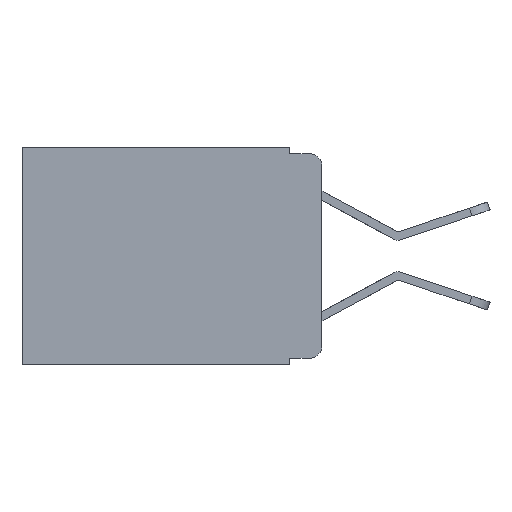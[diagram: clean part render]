
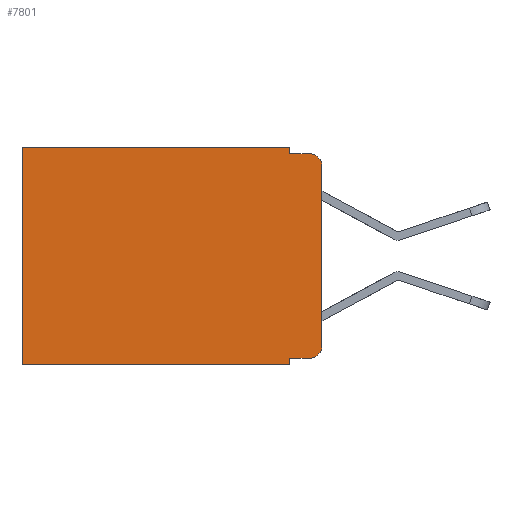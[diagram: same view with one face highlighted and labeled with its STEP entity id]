
A CAD part, left-side view. The second image highlights one B-rep face of the part: STEP entity #7801.
In plain terms, the highlighted planar face has unit normal (-1, 0, 0).
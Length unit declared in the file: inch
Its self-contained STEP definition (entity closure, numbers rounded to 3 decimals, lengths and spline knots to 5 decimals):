
#41 = EDGE_CURVE ( 'NONE', #6747, #13839, #7607, .T. ) ;
#63 = CARTESIAN_POINT ( 'NONE',  ( 0.298, 0.051, -0.01 ) ) ;
#324 = CARTESIAN_POINT ( 'NONE',  ( 0.298, 0.02, -0.333 ) ) ;
#330 = EDGE_LOOP ( 'NONE', ( #10132, #17698, #12927, #10647, #9686, #11313, #15292, #1041, #15936, #714 ) ) ;
#372 = LINE ( 'NONE', #13331, #14365 ) ;
#389 = EDGE_CURVE ( 'NONE', #1333, #15356, #3936, .T. ) ;
#497 = CARTESIAN_POINT ( 'NONE',  ( 0.298, 0.051, -0.343 ) ) ;
#714 = ORIENTED_EDGE ( 'NONE', *, *, #389, .T. ) ;
#875 = VERTEX_POINT ( 'NONE', #497 ) ;
#1041 = ORIENTED_EDGE ( 'NONE', *, *, #13506, .F. ) ;
#1333 = VERTEX_POINT ( 'NONE', #324 ) ;
#1615 = LINE ( 'NONE', #13064, #16016 ) ;
#1883 = LINE ( 'NONE', #7735, #16280 ) ;
#2025 = VECTOR ( 'NONE', #6155, 39.37008 ) ;
#2294 = EDGE_CURVE ( 'NONE', #14530, #1333, #1883, .T. ) ;
#2947 = LINE ( 'NONE', #15879, #2025 ) ;
#3490 = EDGE_CURVE ( 'NONE', #10490, #10364, #11896, .T. ) ;
#3571 = CARTESIAN_POINT ( 'NONE',  ( 0.298, 0., -0.03 ) ) ;
#3912 = VECTOR ( 'NONE', #8870, 39.37008 ) ;
#3936 = CIRCLE ( 'NONE', #10385, 0.02 ) ;
#4143 = VECTOR ( 'NONE', #13033, 39.37008 ) ;
#4738 = DIRECTION ( 'NONE',  ( -1., 0., 0. ) ) ;
#4777 = CARTESIAN_POINT ( 'NONE',  ( 0.298, 0.02, -0.03 ) ) ;
#4855 = CARTESIAN_POINT ( 'NONE',  ( 0.298, 0.473, -0.343 ) ) ;
#5019 = DIRECTION ( 'NONE',  ( 0., 0., -1. ) ) ;
#5023 = CARTESIAN_POINT ( 'NONE',  ( 0.298, 0., -0.313 ) ) ;
#5196 = DIRECTION ( 'NONE',  ( 1., 0., 0. ) ) ;
#6155 = DIRECTION ( 'NONE',  ( 0., 1., 0. ) ) ;
#6409 = CARTESIAN_POINT ( 'NONE',  ( 0.298, 0.473, 0. ) ) ;
#6421 = FACE_OUTER_BOUND ( 'NONE', #330, .T. ) ;
#6747 = VERTEX_POINT ( 'NONE', #14285 ) ;
#7385 = DIRECTION ( 'NONE',  ( 0., 0., -1. ) ) ;
#7607 = LINE ( 'NONE', #10515, #3912 ) ;
#7622 = DIRECTION ( 'NONE',  ( 0., -1., 0. ) ) ;
#7626 = EDGE_CURVE ( 'NONE', #6747, #16490, #2947, .T. ) ;
#7735 = CARTESIAN_POINT ( 'NONE',  ( 0.298, 0.051, -0.333 ) ) ;
#7801 = ADVANCED_FACE ( 'NONE', ( #6421 ), #13512, .F. ) ;
#7842 = LINE ( 'NONE', #8880, #4143 ) ;
#8300 = EDGE_CURVE ( 'NONE', #875, #12266, #16808, .T. ) ;
#8870 = DIRECTION ( 'NONE',  ( 0., 0., -1. ) ) ;
#8880 = CARTESIAN_POINT ( 'NONE',  ( 0.298, 0.051, -0.01 ) ) ;
#9223 = DIRECTION ( 'NONE',  ( 0., 0., -1. ) ) ;
#9313 = LINE ( 'NONE', #6409, #16238 ) ;
#9339 = CARTESIAN_POINT ( 'NONE',  ( 0.298, 0., 0. ) ) ;
#9686 = ORIENTED_EDGE ( 'NONE', *, *, #7626, .T. ) ;
#9743 = CARTESIAN_POINT ( 'NONE',  ( 0.298, 0.473, 0. ) ) ;
#9757 = AXIS2_PLACEMENT_3D ( 'NONE', #9339, #5196, #14919 ) ;
#10132 = ORIENTED_EDGE ( 'NONE', *, *, #15608, .F. ) ;
#10358 = DIRECTION ( 'NONE',  ( -1., 0., 0. ) ) ;
#10364 = VERTEX_POINT ( 'NONE', #11662 ) ;
#10372 = EDGE_CURVE ( 'NONE', #13839, #10364, #7842, .T. ) ;
#10385 = AXIS2_PLACEMENT_3D ( 'NONE', #17068, #10358, #16396 ) ;
#10490 = VERTEX_POINT ( 'NONE', #3571 ) ;
#10515 = CARTESIAN_POINT ( 'NONE',  ( 0.298, 0.051, 0. ) ) ;
#10647 = ORIENTED_EDGE ( 'NONE', *, *, #41, .F. ) ;
#11313 = ORIENTED_EDGE ( 'NONE', *, *, #15384, .T. ) ;
#11662 = CARTESIAN_POINT ( 'NONE',  ( 0.298, 0.02, -0.01 ) ) ;
#11689 = DIRECTION ( 'NONE',  ( 0., 0., -1. ) ) ;
#11896 = CIRCLE ( 'NONE', #15320, 0.02 ) ;
#12266 = VERTEX_POINT ( 'NONE', #4855 ) ;
#12734 = CARTESIAN_POINT ( 'NONE',  ( 0.298, 0.051, -0.333 ) ) ;
#12927 = ORIENTED_EDGE ( 'NONE', *, *, #10372, .F. ) ;
#13033 = DIRECTION ( 'NONE',  ( 0., -1., 0. ) ) ;
#13064 = CARTESIAN_POINT ( 'NONE',  ( 0.298, 0., 0. ) ) ;
#13331 = CARTESIAN_POINT ( 'NONE',  ( 0.298, 0.051, 0. ) ) ;
#13506 = EDGE_CURVE ( 'NONE', #14530, #875, #372, .T. ) ;
#13512 = PLANE ( 'NONE',  #9757 ) ;
#13839 = VERTEX_POINT ( 'NONE', #63 ) ;
#14285 = CARTESIAN_POINT ( 'NONE',  ( 0.298, 0.051, 0. ) ) ;
#14365 = VECTOR ( 'NONE', #5019, 39.37008 ) ;
#14530 = VERTEX_POINT ( 'NONE', #12734 ) ;
#14919 = DIRECTION ( 'NONE',  ( 0., 0., -1. ) ) ;
#15292 = ORIENTED_EDGE ( 'NONE', *, *, #8300, .F. ) ;
#15320 = AXIS2_PLACEMENT_3D ( 'NONE', #4777, #4738, #7385 ) ;
#15356 = VERTEX_POINT ( 'NONE', #5023 ) ;
#15384 = EDGE_CURVE ( 'NONE', #16490, #12266, #9313, .T. ) ;
#15608 = EDGE_CURVE ( 'NONE', #10490, #15356, #1615, .T. ) ;
#15879 = CARTESIAN_POINT ( 'NONE',  ( 0.298, 0., 0. ) ) ;
#15936 = ORIENTED_EDGE ( 'NONE', *, *, #2294, .T. ) ;
#16016 = VECTOR ( 'NONE', #11689, 39.37008 ) ;
#16037 = CARTESIAN_POINT ( 'NONE',  ( 0.298, 0., -0.343 ) ) ;
#16238 = VECTOR ( 'NONE', #9223, 39.37008 ) ;
#16280 = VECTOR ( 'NONE', #7622, 39.37008 ) ;
#16396 = DIRECTION ( 'NONE',  ( 0., 0., -1. ) ) ;
#16490 = VERTEX_POINT ( 'NONE', #9743 ) ;
#16808 = LINE ( 'NONE', #16037, #17666 ) ;
#17068 = CARTESIAN_POINT ( 'NONE',  ( 0.298, 0.02, -0.313 ) ) ;
#17407 = DIRECTION ( 'NONE',  ( 0., 1., 0. ) ) ;
#17666 = VECTOR ( 'NONE', #17407, 39.37008 ) ;
#17698 = ORIENTED_EDGE ( 'NONE', *, *, #3490, .T. ) ;
